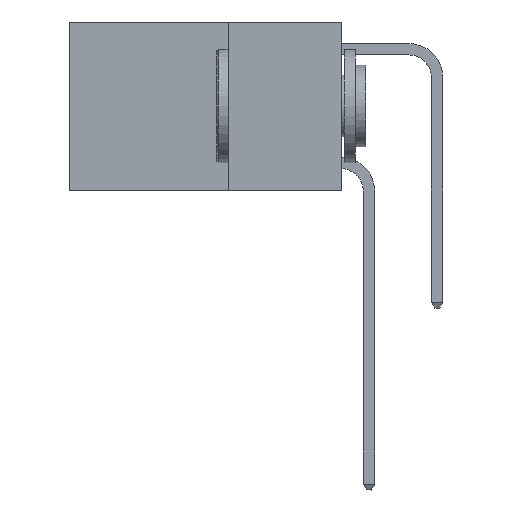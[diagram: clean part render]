
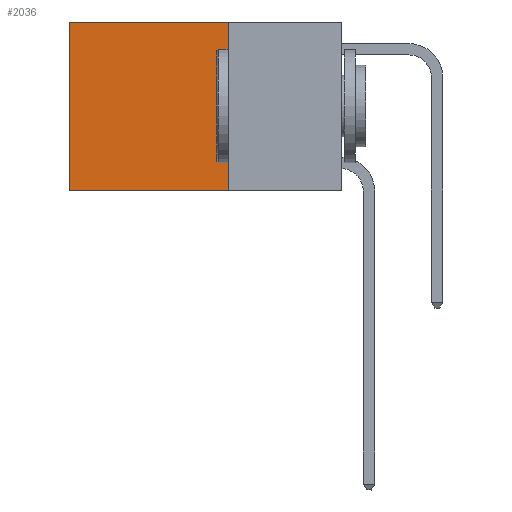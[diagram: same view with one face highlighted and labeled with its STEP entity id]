
A CAD part, left-side view. The second image highlights one B-rep face of the part: STEP entity #2036.
In plain terms, the highlighted planar face has unit normal (-1, 0, 0).
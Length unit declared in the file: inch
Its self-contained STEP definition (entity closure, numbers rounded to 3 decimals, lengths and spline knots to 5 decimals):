
#412 = DIRECTION ( 'NONE',  ( 0., 0., -1. ) ) ;
#427 = DIRECTION ( 'NONE',  ( 1., 0., 0. ) ) ;
#644 = PLANE ( 'NONE',  #7129 ) ;
#664 = CARTESIAN_POINT ( 'NONE',  ( 0.2625, 0.25, 0. ) ) ;
#734 = CARTESIAN_POINT ( 'NONE',  ( 0.2625, 0.25, 0. ) ) ;
#1006 = CARTESIAN_POINT ( 'NONE',  ( 0.2625, 0.6, 0. ) ) ;
#1125 = VECTOR ( 'NONE', #4891, 39.37008 ) ;
#1651 = LINE ( 'NONE', #2974, #11641 ) ;
#2036 = ADVANCED_FACE ( 'NONE', ( #11890 ), #644, .F. ) ;
#2212 = LINE ( 'NONE', #10265, #9561 ) ;
#2974 = CARTESIAN_POINT ( 'NONE',  ( 0.2625, 0.25, 0. ) ) ;
#3077 = CARTESIAN_POINT ( 'NONE',  ( 0.2625, 0.6, -0.37 ) ) ;
#3371 = ORIENTED_EDGE ( 'NONE', *, *, #11517, .F. ) ;
#3497 = VERTEX_POINT ( 'NONE', #3891 ) ;
#3845 = EDGE_LOOP ( 'NONE', ( #5634, #8097, #3371, #8433 ) ) ;
#3882 = LINE ( 'NONE', #734, #1125 ) ;
#3891 = CARTESIAN_POINT ( 'NONE',  ( 0.2625, 0.25, 0. ) ) ;
#4369 = CARTESIAN_POINT ( 'NONE',  ( 0.2625, 0.25, -0.37 ) ) ;
#4891 = DIRECTION ( 'NONE',  ( 0., 1., 0. ) ) ;
#4928 = DIRECTION ( 'NONE',  ( 0., 0., -1. ) ) ;
#5634 = ORIENTED_EDGE ( 'NONE', *, *, #7103, .T. ) ;
#6489 = VERTEX_POINT ( 'NONE', #3077 ) ;
#6566 = VECTOR ( 'NONE', #11966, 39.37008 ) ;
#6912 = EDGE_CURVE ( 'NONE', #12599, #6489, #11345, .T. ) ;
#7103 = EDGE_CURVE ( 'NONE', #12227, #6489, #2212, .T. ) ;
#7129 = AXIS2_PLACEMENT_3D ( 'NONE', #664, #427, #412 ) ;
#8097 = ORIENTED_EDGE ( 'NONE', *, *, #6912, .F. ) ;
#8433 = ORIENTED_EDGE ( 'NONE', *, *, #10734, .T. ) ;
#9561 = VECTOR ( 'NONE', #11239, 39.37008 ) ;
#10265 = CARTESIAN_POINT ( 'NONE',  ( 0.2625, 0.6, 0. ) ) ;
#10317 = CARTESIAN_POINT ( 'NONE',  ( 0.2625, 0.25, -0.37 ) ) ;
#10734 = EDGE_CURVE ( 'NONE', #3497, #12227, #3882, .T. ) ;
#11239 = DIRECTION ( 'NONE',  ( 0., 0., -1. ) ) ;
#11345 = LINE ( 'NONE', #4369, #6566 ) ;
#11517 = EDGE_CURVE ( 'NONE', #3497, #12599, #1651, .T. ) ;
#11641 = VECTOR ( 'NONE', #4928, 39.37008 ) ;
#11890 = FACE_OUTER_BOUND ( 'NONE', #3845, .T. ) ;
#11966 = DIRECTION ( 'NONE',  ( 0., 1., 0. ) ) ;
#12227 = VERTEX_POINT ( 'NONE', #1006 ) ;
#12599 = VERTEX_POINT ( 'NONE', #10317 ) ;
